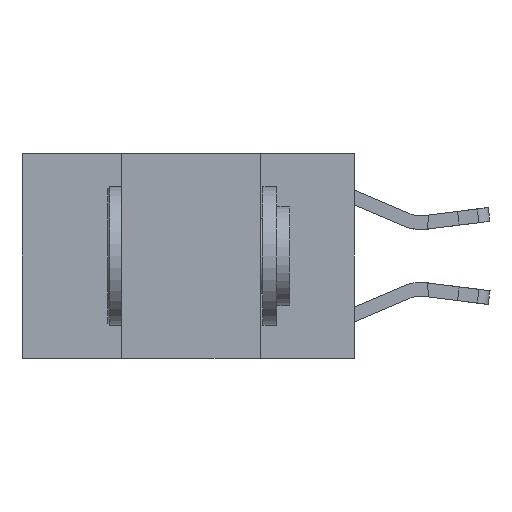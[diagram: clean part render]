
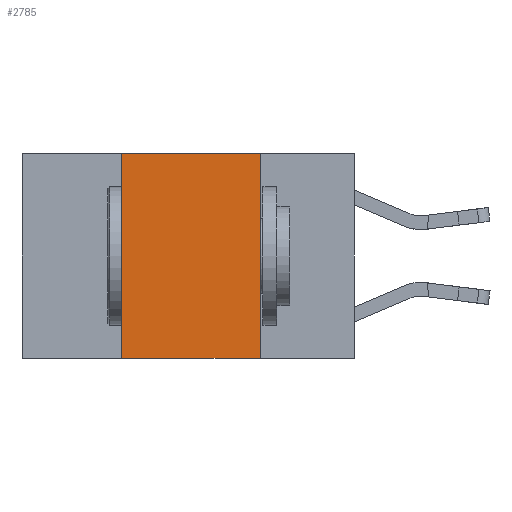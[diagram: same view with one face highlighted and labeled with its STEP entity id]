
A CAD part, left-side view. The second image highlights one B-rep face of the part: STEP entity #2785.
In plain terms, the highlighted planar face has unit normal (-1, 0, 0).
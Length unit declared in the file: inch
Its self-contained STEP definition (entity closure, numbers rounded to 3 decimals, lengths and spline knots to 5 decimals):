
#562 = CARTESIAN_POINT ( 'NONE',  ( 0., 0.17, -0.37 ) ) ;
#688 = EDGE_CURVE ( 'NONE', #1437, #8707, #6036, .T. ) ;
#1168 = DIRECTION ( 'NONE',  ( 0., -1., 0. ) ) ;
#1363 = VECTOR ( 'NONE', #14672, 39.37008 ) ;
#1437 = VERTEX_POINT ( 'NONE', #16918 ) ;
#2721 = EDGE_CURVE ( 'NONE', #7683, #8707, #3131, .T. ) ;
#2785 = ADVANCED_FACE ( 'NONE', ( #5687 ), #12848, .F. ) ;
#3131 = LINE ( 'NONE', #11354, #6576 ) ;
#3361 = DIRECTION ( 'NONE',  ( 0., 0., 1. ) ) ;
#4195 = CARTESIAN_POINT ( 'NONE',  ( 0., 0.42, 0. ) ) ;
#4276 = DIRECTION ( 'NONE',  ( 1., 0., 0. ) ) ;
#4456 = CARTESIAN_POINT ( 'NONE',  ( 0., 0.42, -0.37 ) ) ;
#4920 = CARTESIAN_POINT ( 'NONE',  ( 0., 0.17, 0. ) ) ;
#4982 = DIRECTION ( 'NONE',  ( 0., 0., -1. ) ) ;
#5687 = FACE_OUTER_BOUND ( 'NONE', #8783, .T. ) ;
#6032 = ORIENTED_EDGE ( 'NONE', *, *, #688, .F. ) ;
#6036 = LINE ( 'NONE', #4920, #16516 ) ;
#6576 = VECTOR ( 'NONE', #1168, 39.37008 ) ;
#7092 = CARTESIAN_POINT ( 'NONE',  ( 0., 0.6, 0. ) ) ;
#7683 = VERTEX_POINT ( 'NONE', #4456 ) ;
#8707 = VERTEX_POINT ( 'NONE', #562 ) ;
#8783 = EDGE_LOOP ( 'NONE', ( #6032, #14009, #9651, #14806 ) ) ;
#9139 = LINE ( 'NONE', #13237, #1363 ) ;
#9651 = ORIENTED_EDGE ( 'NONE', *, *, #18470, .F. ) ;
#10442 = AXIS2_PLACEMENT_3D ( 'NONE', #7092, #4276, #14294 ) ;
#10889 = LINE ( 'NONE', #14906, #14255 ) ;
#11354 = CARTESIAN_POINT ( 'NONE',  ( 0., 0.6, -0.37 ) ) ;
#12848 = PLANE ( 'NONE',  #10442 ) ;
#13237 = CARTESIAN_POINT ( 'NONE',  ( 0., 0.6, 0. ) ) ;
#14009 = ORIENTED_EDGE ( 'NONE', *, *, #17620, .F. ) ;
#14255 = VECTOR ( 'NONE', #3361, 39.37008 ) ;
#14294 = DIRECTION ( 'NONE',  ( 0., 0., -1. ) ) ;
#14558 = VERTEX_POINT ( 'NONE', #4195 ) ;
#14672 = DIRECTION ( 'NONE',  ( 0., -1., 0. ) ) ;
#14806 = ORIENTED_EDGE ( 'NONE', *, *, #2721, .T. ) ;
#14906 = CARTESIAN_POINT ( 'NONE',  ( 0., 0.42, 0. ) ) ;
#16516 = VECTOR ( 'NONE', #4982, 39.37008 ) ;
#16918 = CARTESIAN_POINT ( 'NONE',  ( 0., 0.17, 0. ) ) ;
#17620 = EDGE_CURVE ( 'NONE', #14558, #1437, #9139, .T. ) ;
#18470 = EDGE_CURVE ( 'NONE', #7683, #14558, #10889, .T. ) ;
